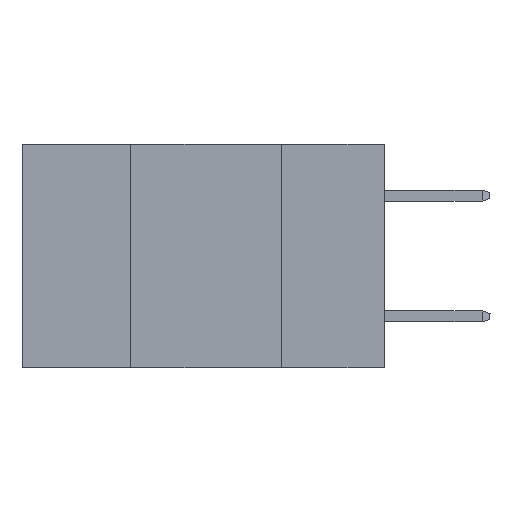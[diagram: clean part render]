
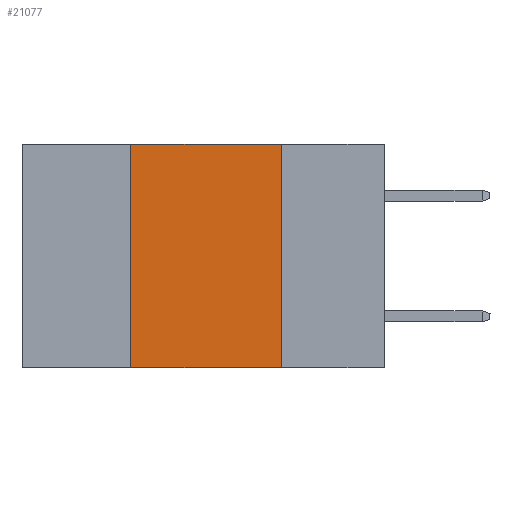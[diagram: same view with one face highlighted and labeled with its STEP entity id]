
A CAD part, left-side view. The second image highlights one B-rep face of the part: STEP entity #21077.
In plain terms, the highlighted planar face has unit normal (-1, 0, 0).
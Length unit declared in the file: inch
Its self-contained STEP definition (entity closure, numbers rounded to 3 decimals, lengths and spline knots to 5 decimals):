
#556 = EDGE_CURVE ( 'NONE', #22049, #25675, #12580, .T. ) ;
#986 = EDGE_LOOP ( 'NONE', ( #1911, #25227, #26847, #23916 ) ) ;
#1911 = ORIENTED_EDGE ( 'NONE', *, *, #556, .F. ) ;
#3257 = LINE ( 'NONE', #15950, #20224 ) ;
#3566 = DIRECTION ( 'NONE',  ( 0., -1., 0. ) ) ;
#4953 = CARTESIAN_POINT ( 'NONE',  ( 0., 0.6, 0. ) ) ;
#6793 = EDGE_CURVE ( 'NONE', #7383, #18721, #3257, .T. ) ;
#7027 = VECTOR ( 'NONE', #3566, 39.37008 ) ;
#7383 = VERTEX_POINT ( 'NONE', #8797 ) ;
#7538 = AXIS2_PLACEMENT_3D ( 'NONE', #4953, #11753, #26704 ) ;
#7867 = DIRECTION ( 'NONE',  ( 0., 0., 1. ) ) ;
#8797 = CARTESIAN_POINT ( 'NONE',  ( 0., 0.42, -0.37 ) ) ;
#9824 = EDGE_CURVE ( 'NONE', #7383, #25675, #18753, .T. ) ;
#10382 = CARTESIAN_POINT ( 'NONE',  ( 0., 0.6, -0.37 ) ) ;
#11753 = DIRECTION ( 'NONE',  ( 1., 0., 0. ) ) ;
#12580 = LINE ( 'NONE', #22965, #17641 ) ;
#13776 = EDGE_CURVE ( 'NONE', #18721, #22049, #20397, .T. ) ;
#14815 = CARTESIAN_POINT ( 'NONE',  ( 0., 0.17, 0. ) ) ;
#15656 = FACE_OUTER_BOUND ( 'NONE', #986, .T. ) ;
#15950 = CARTESIAN_POINT ( 'NONE',  ( 0., 0.42, 0. ) ) ;
#16155 = DIRECTION ( 'NONE',  ( 0., 0., -1. ) ) ;
#17641 = VECTOR ( 'NONE', #16155, 39.37008 ) ;
#18721 = VERTEX_POINT ( 'NONE', #27718 ) ;
#18753 = LINE ( 'NONE', #10382, #7027 ) ;
#19503 = CARTESIAN_POINT ( 'NONE',  ( 0., 0.17, -0.37 ) ) ;
#20224 = VECTOR ( 'NONE', #7867, 39.37008 ) ;
#20397 = LINE ( 'NONE', #23145, #24687 ) ;
#21077 = ADVANCED_FACE ( 'NONE', ( #15656 ), #26604, .F. ) ;
#22049 = VERTEX_POINT ( 'NONE', #14815 ) ;
#22965 = CARTESIAN_POINT ( 'NONE',  ( 0., 0.17, 0. ) ) ;
#23145 = CARTESIAN_POINT ( 'NONE',  ( 0., 0.6, 0. ) ) ;
#23916 = ORIENTED_EDGE ( 'NONE', *, *, #9824, .T. ) ;
#24687 = VECTOR ( 'NONE', #25283, 39.37008 ) ;
#25227 = ORIENTED_EDGE ( 'NONE', *, *, #13776, .F. ) ;
#25283 = DIRECTION ( 'NONE',  ( 0., -1., 0. ) ) ;
#25675 = VERTEX_POINT ( 'NONE', #19503 ) ;
#26604 = PLANE ( 'NONE',  #7538 ) ;
#26704 = DIRECTION ( 'NONE',  ( 0., 0., -1. ) ) ;
#26847 = ORIENTED_EDGE ( 'NONE', *, *, #6793, .F. ) ;
#27718 = CARTESIAN_POINT ( 'NONE',  ( 0., 0.42, 0. ) ) ;
